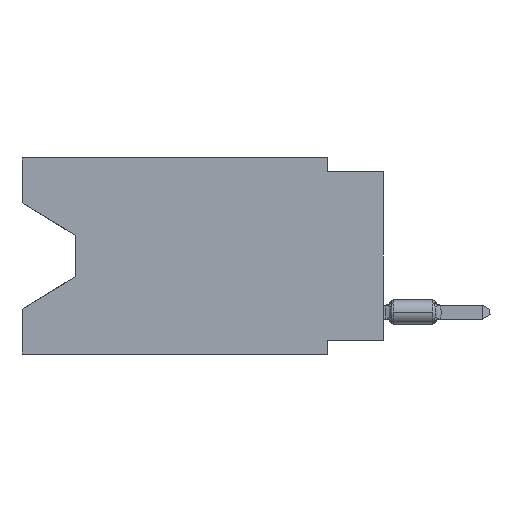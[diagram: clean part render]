
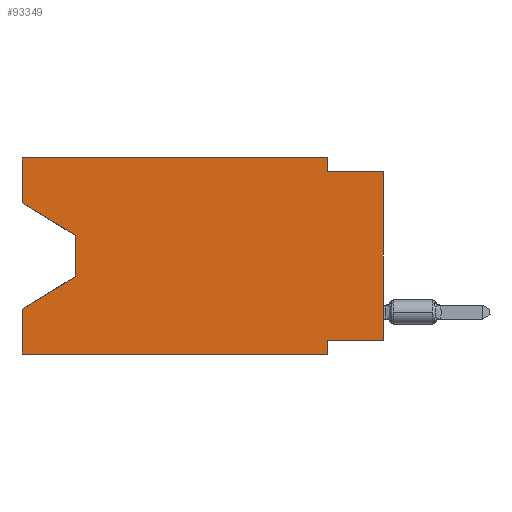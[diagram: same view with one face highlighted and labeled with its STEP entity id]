
A CAD part, left-side view. The second image highlights one B-rep face of the part: STEP entity #93349.
In plain terms, the highlighted planar face has unit normal (-1, 0, 0).
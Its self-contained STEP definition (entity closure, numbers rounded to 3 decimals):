
#11 = EDGE_CURVE ( 'NONE', #70782, #90059, #62175, .T. ) ;
#46 = VERTEX_POINT ( 'NONE', #87197 ) ;
#112 = DIRECTION ( 'NONE',  ( 0., 1., 0. ) ) ;
#277 = DIRECTION ( 'NONE',  ( 0., -1., 0. ) ) ;
#576 = LINE ( 'NONE', #72513, #61001 ) ;
#3205 = EDGE_CURVE ( 'NONE', #72320, #46, #576, .T. ) ;
#3951 = ORIENTED_EDGE ( 'NONE', *, *, #38144, .T. ) ;
#4856 = CARTESIAN_POINT ( 'NONE',  ( 0., 0., -8.255 ) ) ;
#5158 = CARTESIAN_POINT ( 'NONE',  ( 0., 16.383, -8.89 ) ) ;
#5161 = ORIENTED_EDGE ( 'NONE', *, *, #54534, .T. ) ;
#5803 = CARTESIAN_POINT ( 'NONE',  ( 0., 13.97, -5.385 ) ) ;
#7534 = FACE_OUTER_BOUND ( 'NONE', #82551, .T. ) ;
#7671 = DIRECTION ( 'NONE',  ( 0., 0., -1. ) ) ;
#7814 = VECTOR ( 'NONE', #65862, 1000. ) ;
#8946 = ORIENTED_EDGE ( 'NONE', *, *, #63324, .T. ) ;
#9280 = VERTEX_POINT ( 'NONE', #84819 ) ;
#9556 = VECTOR ( 'NONE', #14492, 1000. ) ;
#9731 = CARTESIAN_POINT ( 'NONE',  ( 0., 13.97, -3.505 ) ) ;
#10347 = DIRECTION ( 'NONE',  ( 0., 0., -1. ) ) ;
#11617 = VECTOR ( 'NONE', #74096, 1000. ) ;
#13517 = LINE ( 'NONE', #23775, #21513 ) ;
#13889 = CARTESIAN_POINT ( 'NONE',  ( 0., 13.97, -5.385 ) ) ;
#14492 = DIRECTION ( 'NONE',  ( 0., -1., 0. ) ) ;
#14502 = VECTOR ( 'NONE', #34673, 1000. ) ;
#15891 = LINE ( 'NONE', #37167, #11617 ) ;
#16752 = ORIENTED_EDGE ( 'NONE', *, *, #56706, .F. ) ;
#17304 = DIRECTION ( 'NONE',  ( 0., 0., -1. ) ) ;
#19556 = LINE ( 'NONE', #5803, #14502 ) ;
#19605 = ORIENTED_EDGE ( 'NONE', *, *, #11, .F. ) ;
#21513 = VECTOR ( 'NONE', #72158, 1000. ) ;
#23775 = CARTESIAN_POINT ( 'NONE',  ( 0., 16.383, -8.89 ) ) ;
#24214 = CARTESIAN_POINT ( 'NONE',  ( 0., 2.54, -8.89 ) ) ;
#26221 = CARTESIAN_POINT ( 'NONE',  ( 0., 16.383, 0. ) ) ;
#26697 = LINE ( 'NONE', #29919, #79847 ) ;
#27041 = VERTEX_POINT ( 'NONE', #39570 ) ;
#29100 = VERTEX_POINT ( 'NONE', #4856 ) ;
#29919 = CARTESIAN_POINT ( 'NONE',  ( 0., 0., -8.255 ) ) ;
#30573 = CARTESIAN_POINT ( 'NONE',  ( 0., 2.54, -8.89 ) ) ;
#34673 = DIRECTION ( 'NONE',  ( 0., 0.855, -0.519 ) ) ;
#35127 = VERTEX_POINT ( 'NONE', #30573 ) ;
#36248 = CARTESIAN_POINT ( 'NONE',  ( 0., 0., -0.635 ) ) ;
#37167 = CARTESIAN_POINT ( 'NONE',  ( 0., 16.383, 0. ) ) ;
#37428 = EDGE_CURVE ( 'NONE', #41689, #72320, #42416, .T. ) ;
#37439 = VECTOR ( 'NONE', #77300, 1000. ) ;
#37448 = ORIENTED_EDGE ( 'NONE', *, *, #3205, .F. ) ;
#37679 = CARTESIAN_POINT ( 'NONE',  ( 0., 2.54, -8.255 ) ) ;
#38144 = EDGE_CURVE ( 'NONE', #29100, #9280, #40710, .T. ) ;
#39570 = CARTESIAN_POINT ( 'NONE',  ( 0., 16.383, -2.038 ) ) ;
#40710 = LINE ( 'NONE', #77596, #61025 ) ;
#40880 = ORIENTED_EDGE ( 'NONE', *, *, #55560, .F. ) ;
#41689 = VERTEX_POINT ( 'NONE', #92595 ) ;
#42416 = LINE ( 'NONE', #70829, #9556 ) ;
#43025 = ORIENTED_EDGE ( 'NONE', *, *, #71267, .F. ) ;
#43698 = VECTOR ( 'NONE', #17304, 1000. ) ;
#46531 = VECTOR ( 'NONE', #277, 1000. ) ;
#48724 = DIRECTION ( 'NONE',  ( 0., 0., 1. ) ) ;
#51104 = ORIENTED_EDGE ( 'NONE', *, *, #64524, .T. ) ;
#51344 = LINE ( 'NONE', #56591, #65548 ) ;
#51835 = LINE ( 'NONE', #9731, #43698 ) ;
#53404 = PLANE ( 'NONE',  #82157 ) ;
#53741 = VERTEX_POINT ( 'NONE', #37679 ) ;
#54534 = EDGE_CURVE ( 'NONE', #88251, #90059, #19556, .T. ) ;
#55560 = EDGE_CURVE ( 'NONE', #27041, #41689, #15891, .T. ) ;
#56310 = CARTESIAN_POINT ( 'NONE',  ( 0., 13.97, -3.505 ) ) ;
#56591 = CARTESIAN_POINT ( 'NONE',  ( 0., 16.383, -2.038 ) ) ;
#56706 = EDGE_CURVE ( 'NONE', #46, #9280, #93526, .T. ) ;
#61001 = VECTOR ( 'NONE', #7671, 1000. ) ;
#61025 = VECTOR ( 'NONE', #48724, 1000. ) ;
#62175 = LINE ( 'NONE', #26221, #37439 ) ;
#63324 = EDGE_CURVE ( 'NONE', #70782, #35127, #13517, .T. ) ;
#63370 = ORIENTED_EDGE ( 'NONE', *, *, #37428, .F. ) ;
#63783 = ORIENTED_EDGE ( 'NONE', *, *, #86166, .F. ) ;
#64524 = EDGE_CURVE ( 'NONE', #27041, #81631, #51344, .T. ) ;
#65548 = VECTOR ( 'NONE', #78347, 1000. ) ;
#65862 = DIRECTION ( 'NONE',  ( 0., 0., -1. ) ) ;
#67615 = DIRECTION ( 'NONE',  ( 1., 0., 0. ) ) ;
#70782 = VERTEX_POINT ( 'NONE', #5158 ) ;
#70829 = CARTESIAN_POINT ( 'NONE',  ( 0., 16.383, 0. ) ) ;
#71267 = EDGE_CURVE ( 'NONE', #29100, #53741, #26697, .T. ) ;
#72158 = DIRECTION ( 'NONE',  ( 0., -1., 0. ) ) ;
#72320 = VERTEX_POINT ( 'NONE', #74658 ) ;
#72513 = CARTESIAN_POINT ( 'NONE',  ( 0., 2.54, 0. ) ) ;
#74089 = EDGE_CURVE ( 'NONE', #81631, #88251, #51835, .T. ) ;
#74096 = DIRECTION ( 'NONE',  ( 0., 0., 1. ) ) ;
#74658 = CARTESIAN_POINT ( 'NONE',  ( 0., 2.54, 0. ) ) ;
#75183 = CARTESIAN_POINT ( 'NONE',  ( 0., 16.383, 0. ) ) ;
#75418 = ORIENTED_EDGE ( 'NONE', *, *, #74089, .T. ) ;
#77300 = DIRECTION ( 'NONE',  ( 0., 0., 1. ) ) ;
#77596 = CARTESIAN_POINT ( 'NONE',  ( 0., 0., 0. ) ) ;
#78347 = DIRECTION ( 'NONE',  ( 0., -0.855, -0.519 ) ) ;
#79847 = VECTOR ( 'NONE', #112, 1000. ) ;
#80048 = LINE ( 'NONE', #24214, #7814 ) ;
#81631 = VERTEX_POINT ( 'NONE', #56310 ) ;
#82157 = AXIS2_PLACEMENT_3D ( 'NONE', #75183, #67615, #10347 ) ;
#82551 = EDGE_LOOP ( 'NONE', ( #51104, #75418, #5161, #19605, #8946, #63783, #43025, #3951, #16752, #37448, #63370, #40880 ) ) ;
#84198 = CARTESIAN_POINT ( 'NONE',  ( 0., 16.383, -6.852 ) ) ;
#84819 = CARTESIAN_POINT ( 'NONE',  ( 0., 0., -0.635 ) ) ;
#86166 = EDGE_CURVE ( 'NONE', #53741, #35127, #80048, .T. ) ;
#87197 = CARTESIAN_POINT ( 'NONE',  ( 0., 2.54, -0.635 ) ) ;
#88251 = VERTEX_POINT ( 'NONE', #13889 ) ;
#90059 = VERTEX_POINT ( 'NONE', #84198 ) ;
#92595 = CARTESIAN_POINT ( 'NONE',  ( 0., 16.383, 0. ) ) ;
#93349 = ADVANCED_FACE ( 'NONE', ( #7534 ), #53404, .F. ) ;
#93526 = LINE ( 'NONE', #36248, #46531 ) ;
